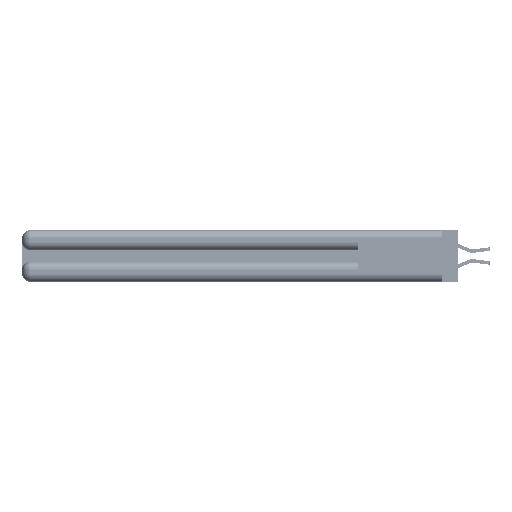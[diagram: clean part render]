
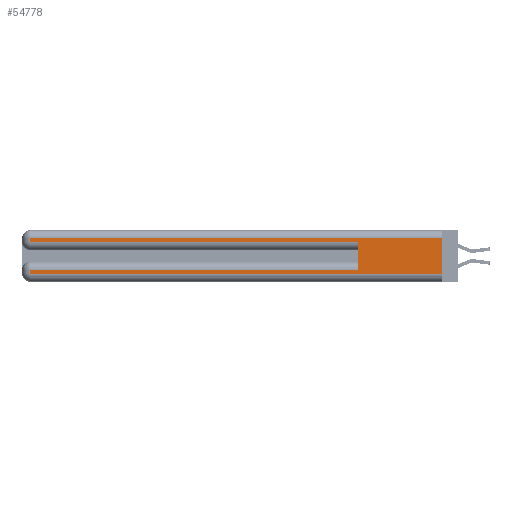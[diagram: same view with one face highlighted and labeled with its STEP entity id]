
A CAD part, left-side view. The second image highlights one B-rep face of the part: STEP entity #54778.
In plain terms, the highlighted planar face has unit normal (-1, 0, 0).
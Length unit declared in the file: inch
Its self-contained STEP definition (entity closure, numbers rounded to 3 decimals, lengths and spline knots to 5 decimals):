
#279 = VERTEX_POINT ( 'NONE', #24356 ) ;
#306 = VECTOR ( 'NONE', #22304, 39.37008 ) ;
#2010 = CARTESIAN_POINT ( 'NONE',  ( 0., 2.94, 0.37 ) ) ;
#2723 = CARTESIAN_POINT ( 'NONE',  ( 0., 2.94, 0.37 ) ) ;
#2786 = ORIENTED_EDGE ( 'NONE', *, *, #15054, .T. ) ;
#2866 = LINE ( 'NONE', #29596, #35237 ) ;
#3219 = VERTEX_POINT ( 'NONE', #43242 ) ;
#6404 = VECTOR ( 'NONE', #10349, 39.37008 ) ;
#6555 = CARTESIAN_POINT ( 'NONE',  ( 0., 2.94, 0.31 ) ) ;
#7283 = AXIS2_PLACEMENT_3D ( 'NONE', #50458, #54740, #29278 ) ;
#8277 = FACE_OUTER_BOUND ( 'NONE', #22428, .T. ) ;
#9365 = VERTEX_POINT ( 'NONE', #23963 ) ;
#9689 = ORIENTED_EDGE ( 'NONE', *, *, #15065, .T. ) ;
#10349 = DIRECTION ( 'NONE',  ( 0., 0., -1. ) ) ;
#12970 = LINE ( 'NONE', #30473, #34085 ) ;
#13307 = CARTESIAN_POINT ( 'NONE',  ( 0., 2.94, 0.085 ) ) ;
#13544 = EDGE_CURVE ( 'NONE', #45069, #46897, #2866, .T. ) ;
#14559 = VECTOR ( 'NONE', #15462, 39.37008 ) ;
#14868 = LINE ( 'NONE', #15683, #24771 ) ;
#15054 = EDGE_CURVE ( 'NONE', #45069, #50463, #49690, .T. ) ;
#15065 = EDGE_CURVE ( 'NONE', #23648, #9365, #25759, .T. ) ;
#15277 = CARTESIAN_POINT ( 'NONE',  ( 0., 0., 0.085 ) ) ;
#15462 = DIRECTION ( 'NONE',  ( 0., 0., -1. ) ) ;
#15683 = CARTESIAN_POINT ( 'NONE',  ( 0., 0., 0.285 ) ) ;
#15891 = VECTOR ( 'NONE', #53283, 39.37008 ) ;
#16854 = CARTESIAN_POINT ( 'NONE',  ( 0., 0., 0.31 ) ) ;
#20780 = PLANE ( 'NONE',  #7283 ) ;
#22304 = DIRECTION ( 'NONE',  ( 0., -1., 0. ) ) ;
#22428 = EDGE_LOOP ( 'NONE', ( #54220, #39211, #9689, #46167, #42875, #2786, #50175, #41514 ) ) ;
#23648 = VERTEX_POINT ( 'NONE', #6555 ) ;
#23963 = CARTESIAN_POINT ( 'NONE',  ( 0., 2.94, 0.285 ) ) ;
#24067 = LINE ( 'NONE', #47484, #35329 ) ;
#24354 = EDGE_CURVE ( 'NONE', #25463, #3219, #24067, .T. ) ;
#24356 = CARTESIAN_POINT ( 'NONE',  ( 0., 2.94, 0.06 ) ) ;
#24771 = VECTOR ( 'NONE', #36755, 39.37008 ) ;
#25463 = VERTEX_POINT ( 'NONE', #16854 ) ;
#25759 = LINE ( 'NONE', #2723, #14559 ) ;
#29278 = DIRECTION ( 'NONE',  ( 0., 0., -1. ) ) ;
#29505 = EDGE_CURVE ( 'NONE', #50463, #279, #40121, .T. ) ;
#29596 = CARTESIAN_POINT ( 'NONE',  ( 0., 0.6, 0.145 ) ) ;
#30473 = CARTESIAN_POINT ( 'NONE',  ( 0., 0., 0.31 ) ) ;
#30616 = CARTESIAN_POINT ( 'NONE',  ( 0., 0., 0.06 ) ) ;
#34085 = VECTOR ( 'NONE', #47533, 39.37008 ) ;
#35237 = VECTOR ( 'NONE', #38110, 39.37008 ) ;
#35329 = VECTOR ( 'NONE', #51807, 39.37008 ) ;
#35383 = LINE ( 'NONE', #30616, #306 ) ;
#36755 = DIRECTION ( 'NONE',  ( 0., -1., 0. ) ) ;
#38110 = DIRECTION ( 'NONE',  ( 0., 0., 1. ) ) ;
#39022 = EDGE_CURVE ( 'NONE', #25463, #23648, #12970, .T. ) ;
#39211 = ORIENTED_EDGE ( 'NONE', *, *, #39022, .T. ) ;
#39565 = EDGE_CURVE ( 'NONE', #279, #3219, #35383, .T. ) ;
#39855 = CARTESIAN_POINT ( 'NONE',  ( 0., 0.6, 0.285 ) ) ;
#40121 = LINE ( 'NONE', #2010, #6404 ) ;
#40227 = CARTESIAN_POINT ( 'NONE',  ( 0., 0.6, 0.085 ) ) ;
#41514 = ORIENTED_EDGE ( 'NONE', *, *, #39565, .T. ) ;
#42875 = ORIENTED_EDGE ( 'NONE', *, *, #13544, .F. ) ;
#43242 = CARTESIAN_POINT ( 'NONE',  ( 0., 0., 0.06 ) ) ;
#45069 = VERTEX_POINT ( 'NONE', #40227 ) ;
#46167 = ORIENTED_EDGE ( 'NONE', *, *, #48891, .T. ) ;
#46897 = VERTEX_POINT ( 'NONE', #39855 ) ;
#47484 = CARTESIAN_POINT ( 'NONE',  ( 0., 0., 0.37 ) ) ;
#47533 = DIRECTION ( 'NONE',  ( 0., 1., 0. ) ) ;
#48891 = EDGE_CURVE ( 'NONE', #9365, #46897, #14868, .T. ) ;
#49690 = LINE ( 'NONE', #15277, #15891 ) ;
#50175 = ORIENTED_EDGE ( 'NONE', *, *, #29505, .T. ) ;
#50458 = CARTESIAN_POINT ( 'NONE',  ( 0., 0., 0.37 ) ) ;
#50463 = VERTEX_POINT ( 'NONE', #13307 ) ;
#51807 = DIRECTION ( 'NONE',  ( 0., 0., -1. ) ) ;
#53283 = DIRECTION ( 'NONE',  ( 0., 1., 0. ) ) ;
#54220 = ORIENTED_EDGE ( 'NONE', *, *, #24354, .F. ) ;
#54740 = DIRECTION ( 'NONE',  ( 1., 0., 0. ) ) ;
#54778 = ADVANCED_FACE ( 'NONE', ( #8277 ), #20780, .F. ) ;
